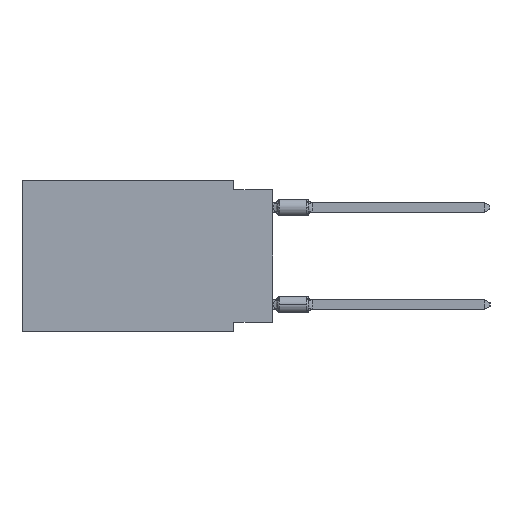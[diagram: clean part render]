
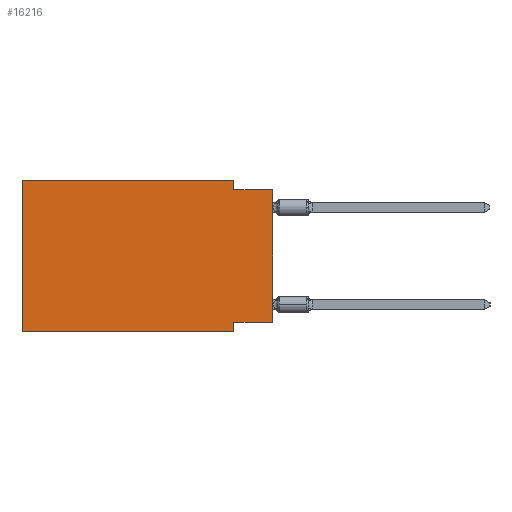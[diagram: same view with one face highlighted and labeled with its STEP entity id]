
A CAD part, left-side view. The second image highlights one B-rep face of the part: STEP entity #16216.
In plain terms, the highlighted planar face has unit normal (-1, 0, 0).
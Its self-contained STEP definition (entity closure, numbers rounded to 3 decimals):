
#938 = DIRECTION ( 'NONE',  ( 0., -1., 0. ) ) ;
#1355 = CARTESIAN_POINT ( 'NONE',  ( 0., 16.383, 0. ) ) ;
#1934 = DIRECTION ( 'NONE',  ( 0., 0., 1. ) ) ;
#2160 = CARTESIAN_POINT ( 'NONE',  ( 0., 2.54, -0.635 ) ) ;
#2176 = LINE ( 'NONE', #27620, #6886 ) ;
#3151 = ORIENTED_EDGE ( 'NONE', *, *, #15502, .F. ) ;
#3600 = VECTOR ( 'NONE', #938, 1000. ) ;
#3750 = CARTESIAN_POINT ( 'NONE',  ( 0., 0., -9.271 ) ) ;
#3843 = VECTOR ( 'NONE', #7902, 1000. ) ;
#4306 = VERTEX_POINT ( 'NONE', #17068 ) ;
#5038 = LINE ( 'NONE', #7449, #3843 ) ;
#5691 = CARTESIAN_POINT ( 'NONE',  ( 0., 2.54, 0. ) ) ;
#5852 = CARTESIAN_POINT ( 'NONE',  ( 0., 2.54, -9.906 ) ) ;
#5854 = VERTEX_POINT ( 'NONE', #15885 ) ;
#6619 = LINE ( 'NONE', #15796, #11175 ) ;
#6886 = VECTOR ( 'NONE', #16179, 1000. ) ;
#7449 = CARTESIAN_POINT ( 'NONE',  ( 0., 0., -0.635 ) ) ;
#7902 = DIRECTION ( 'NONE',  ( 0., -1., 0. ) ) ;
#8737 = DIRECTION ( 'NONE',  ( 0., 1., 0. ) ) ;
#9293 = EDGE_CURVE ( 'NONE', #29558, #12034, #5038, .T. ) ;
#10023 = ORIENTED_EDGE ( 'NONE', *, *, #19175, .F. ) ;
#10156 = CARTESIAN_POINT ( 'NONE',  ( 0., 16.383, -9.906 ) ) ;
#10508 = EDGE_CURVE ( 'NONE', #5854, #23868, #20176, .T. ) ;
#11175 = VECTOR ( 'NONE', #1934, 1000. ) ;
#11734 = ORIENTED_EDGE ( 'NONE', *, *, #20239, .F. ) ;
#11977 = EDGE_CURVE ( 'NONE', #4306, #29558, #26173, .T. ) ;
#12034 = VERTEX_POINT ( 'NONE', #21509 ) ;
#12934 = EDGE_CURVE ( 'NONE', #29240, #29061, #23708, .T. ) ;
#13871 = VERTEX_POINT ( 'NONE', #23742 ) ;
#14367 = DIRECTION ( 'NONE',  ( 0., 0., 1. ) ) ;
#14927 = PLANE ( 'NONE',  #19359 ) ;
#15034 = DIRECTION ( 'NONE',  ( 0., 0., -1. ) ) ;
#15502 = EDGE_CURVE ( 'NONE', #13871, #4306, #22532, .T. ) ;
#15526 = DIRECTION ( 'NONE',  ( 0., 0., -1. ) ) ;
#15796 = CARTESIAN_POINT ( 'NONE',  ( 0., 16.383, 0. ) ) ;
#15885 = CARTESIAN_POINT ( 'NONE',  ( 0., 0., -9.271 ) ) ;
#16179 = DIRECTION ( 'NONE',  ( 0., 0., -1. ) ) ;
#16196 = DIRECTION ( 'NONE',  ( 0., -1., 0. ) ) ;
#16216 = ADVANCED_FACE ( 'NONE', ( #22004 ), #14927, .F. ) ;
#16485 = CARTESIAN_POINT ( 'NONE',  ( 0., 0., 0. ) ) ;
#16628 = LINE ( 'NONE', #16485, #19892 ) ;
#17068 = CARTESIAN_POINT ( 'NONE',  ( 0., 2.54, 0. ) ) ;
#18908 = VECTOR ( 'NONE', #15034, 1000. ) ;
#19175 = EDGE_CURVE ( 'NONE', #29240, #13871, #6619, .T. ) ;
#19359 = AXIS2_PLACEMENT_3D ( 'NONE', #1355, #24262, #15526 ) ;
#19892 = VECTOR ( 'NONE', #14367, 1000. ) ;
#20176 = LINE ( 'NONE', #3750, #29031 ) ;
#20239 = EDGE_CURVE ( 'NONE', #23868, #29061, #2176, .T. ) ;
#20874 = CARTESIAN_POINT ( 'NONE',  ( 0., 16.383, -9.906 ) ) ;
#21509 = CARTESIAN_POINT ( 'NONE',  ( 0., 0., -0.635 ) ) ;
#22004 = FACE_OUTER_BOUND ( 'NONE', #24532, .T. ) ;
#22217 = ORIENTED_EDGE ( 'NONE', *, *, #28085, .T. ) ;
#22532 = LINE ( 'NONE', #27636, #27758 ) ;
#23708 = LINE ( 'NONE', #10156, #3600 ) ;
#23742 = CARTESIAN_POINT ( 'NONE',  ( 0., 16.383, 0. ) ) ;
#23868 = VERTEX_POINT ( 'NONE', #25360 ) ;
#24262 = DIRECTION ( 'NONE',  ( 1., 0., 0. ) ) ;
#24532 = EDGE_LOOP ( 'NONE', ( #22217, #25056, #25812, #3151, #10023, #27754, #11734, #25606 ) ) ;
#25056 = ORIENTED_EDGE ( 'NONE', *, *, #9293, .F. ) ;
#25360 = CARTESIAN_POINT ( 'NONE',  ( 0., 2.54, -9.271 ) ) ;
#25606 = ORIENTED_EDGE ( 'NONE', *, *, #10508, .F. ) ;
#25812 = ORIENTED_EDGE ( 'NONE', *, *, #11977, .F. ) ;
#26173 = LINE ( 'NONE', #5691, #18908 ) ;
#27620 = CARTESIAN_POINT ( 'NONE',  ( 0., 2.54, -9.906 ) ) ;
#27636 = CARTESIAN_POINT ( 'NONE',  ( 0., 16.383, 0. ) ) ;
#27754 = ORIENTED_EDGE ( 'NONE', *, *, #12934, .T. ) ;
#27758 = VECTOR ( 'NONE', #16196, 1000. ) ;
#28085 = EDGE_CURVE ( 'NONE', #5854, #12034, #16628, .T. ) ;
#29031 = VECTOR ( 'NONE', #8737, 1000. ) ;
#29061 = VERTEX_POINT ( 'NONE', #5852 ) ;
#29240 = VERTEX_POINT ( 'NONE', #20874 ) ;
#29558 = VERTEX_POINT ( 'NONE', #2160 ) ;
